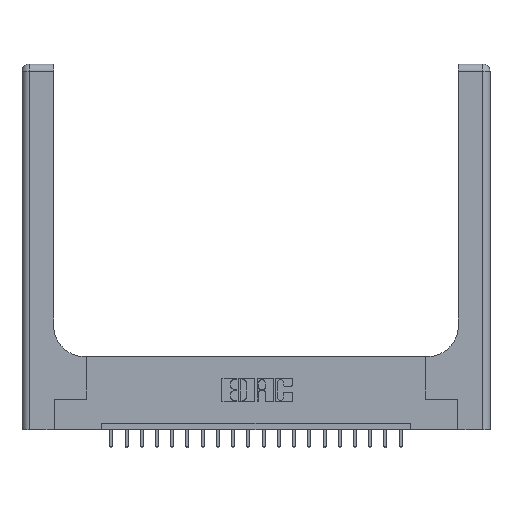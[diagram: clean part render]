
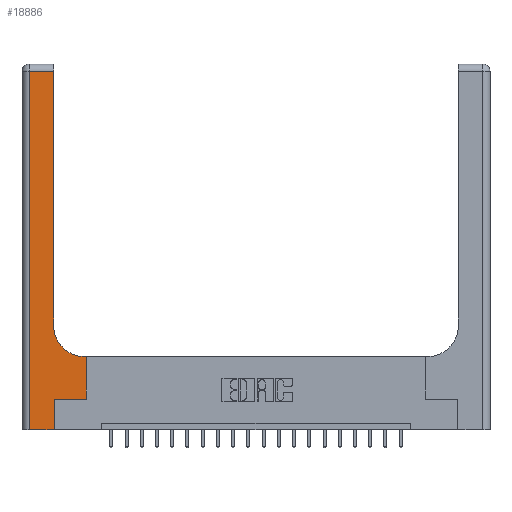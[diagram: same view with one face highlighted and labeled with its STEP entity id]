
A CAD part, top view. The second image highlights one B-rep face of the part: STEP entity #18886.
In plain terms, the highlighted planar face has unit normal (0, 0, 1).
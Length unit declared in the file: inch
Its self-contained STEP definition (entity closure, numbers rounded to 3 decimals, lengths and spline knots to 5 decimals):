
#230 = DIRECTION ( 'NONE',  ( 0., 1., 0. ) ) ;
#360 = CARTESIAN_POINT ( 'NONE',  ( 0.528, 0.25, 0.37 ) ) ;
#778 = VERTEX_POINT ( 'NONE', #14954 ) ;
#841 = DIRECTION ( 'NONE',  ( -1., 0., 0. ) ) ;
#962 = CARTESIAN_POINT ( 'NONE',  ( 0.06, 2.94, 0.37 ) ) ;
#1283 = CARTESIAN_POINT ( 'NONE',  ( 0.26, 0.85, 0.37 ) ) ;
#1516 = ORIENTED_EDGE ( 'NONE', *, *, #11680, .T. ) ;
#2709 = ORIENTED_EDGE ( 'NONE', *, *, #11564, .T. ) ;
#3017 = DIRECTION ( 'NONE',  ( 0., 1., 0. ) ) ;
#3072 = VECTOR ( 'NONE', #16020, 39.37008 ) ;
#3203 = VECTOR ( 'NONE', #3858, 39.37008 ) ;
#3858 = DIRECTION ( 'NONE',  ( 1., 0., 0. ) ) ;
#3915 = CARTESIAN_POINT ( 'NONE',  ( 0.528, 0.25, 0.37 ) ) ;
#4223 = CARTESIAN_POINT ( 'NONE',  ( 0.51, 0.6, 0.37 ) ) ;
#4250 = VERTEX_POINT ( 'NONE', #11984 ) ;
#5029 = DIRECTION ( 'NONE',  ( 0., -1., 0. ) ) ;
#6157 = LINE ( 'NONE', #360, #13315 ) ;
#6390 = VERTEX_POINT ( 'NONE', #7129 ) ;
#6578 = EDGE_CURVE ( 'NONE', #778, #15847, #7678, .T. ) ;
#6653 = CARTESIAN_POINT ( 'NONE',  ( 0.06, 3., 0.37 ) ) ;
#6901 = EDGE_CURVE ( 'NONE', #19575, #14917, #12826, .T. ) ;
#7124 = VECTOR ( 'NONE', #17889, 39.37008 ) ;
#7129 = CARTESIAN_POINT ( 'NONE',  ( 0.265, 0., 0.37 ) ) ;
#7236 = DIRECTION ( 'NONE',  ( 0., 0., -1. ) ) ;
#7390 = AXIS2_PLACEMENT_3D ( 'NONE', #13699, #7236, #7747 ) ;
#7492 = CARTESIAN_POINT ( 'NONE',  ( 0.265, 0., 0.37 ) ) ;
#7678 = LINE ( 'NONE', #18283, #3203 ) ;
#7747 = DIRECTION ( 'NONE',  ( 1., 0., 0. ) ) ;
#8432 = DIRECTION ( 'NONE',  ( 1., 0., 0. ) ) ;
#8637 = CARTESIAN_POINT ( 'NONE',  ( 0., 3., 0.37 ) ) ;
#8917 = EDGE_CURVE ( 'NONE', #13680, #4250, #11285, .T. ) ;
#9224 = VERTEX_POINT ( 'NONE', #9967 ) ;
#9354 = ORIENTED_EDGE ( 'NONE', *, *, #14168, .T. ) ;
#9626 = CARTESIAN_POINT ( 'NONE',  ( 0.26, 2.94, 0.37 ) ) ;
#9837 = ORIENTED_EDGE ( 'NONE', *, *, #8917, .T. ) ;
#9905 = ORIENTED_EDGE ( 'NONE', *, *, #17440, .T. ) ;
#9967 = CARTESIAN_POINT ( 'NONE',  ( 0.528, 0.6, 0.37 ) ) ;
#10087 = LINE ( 'NONE', #14946, #15532 ) ;
#10272 = ORIENTED_EDGE ( 'NONE', *, *, #12328, .T. ) ;
#10383 = DIRECTION ( 'NONE',  ( 0., 0., -1. ) ) ;
#11285 = LINE ( 'NONE', #6653, #20509 ) ;
#11452 = ORIENTED_EDGE ( 'NONE', *, *, #6901, .T. ) ;
#11564 = EDGE_CURVE ( 'NONE', #6390, #778, #12114, .T. ) ;
#11675 = PLANE ( 'NONE',  #18309 ) ;
#11680 = EDGE_CURVE ( 'NONE', #15847, #9224, #6157, .T. ) ;
#11927 = CIRCLE ( 'NONE', #7390, 0.25 ) ;
#11984 = CARTESIAN_POINT ( 'NONE',  ( 0.06, 0., 0.37 ) ) ;
#12114 = LINE ( 'NONE', #7492, #7124 ) ;
#12231 = EDGE_LOOP ( 'NONE', ( #11452, #9354, #9837, #10272, #2709, #13361, #1516, #9905, #14223 ) ) ;
#12328 = EDGE_CURVE ( 'NONE', #4250, #6390, #10087, .T. ) ;
#12357 = VECTOR ( 'NONE', #3017, 39.37008 ) ;
#12713 = LINE ( 'NONE', #20363, #3072 ) ;
#12826 = LINE ( 'NONE', #18957, #12357 ) ;
#12957 = LINE ( 'NONE', #13297, #13450 ) ;
#13297 = CARTESIAN_POINT ( 'NONE',  ( 0.26, 0.6, 0.37 ) ) ;
#13315 = VECTOR ( 'NONE', #230, 39.37008 ) ;
#13361 = ORIENTED_EDGE ( 'NONE', *, *, #6578, .T. ) ;
#13450 = VECTOR ( 'NONE', #841, 39.37008 ) ;
#13680 = VERTEX_POINT ( 'NONE', #962 ) ;
#13699 = CARTESIAN_POINT ( 'NONE',  ( 0.51, 0.85, 0.37 ) ) ;
#14168 = EDGE_CURVE ( 'NONE', #14917, #13680, #12713, .T. ) ;
#14223 = ORIENTED_EDGE ( 'NONE', *, *, #18960, .T. ) ;
#14917 = VERTEX_POINT ( 'NONE', #9626 ) ;
#14946 = CARTESIAN_POINT ( 'NONE',  ( 0., 0., 0.37 ) ) ;
#14954 = CARTESIAN_POINT ( 'NONE',  ( 0.265, 0.25, 0.37 ) ) ;
#15361 = VERTEX_POINT ( 'NONE', #4223 ) ;
#15532 = VECTOR ( 'NONE', #8432, 39.37008 ) ;
#15847 = VERTEX_POINT ( 'NONE', #3915 ) ;
#16020 = DIRECTION ( 'NONE',  ( -1., 0., 0. ) ) ;
#16522 = DIRECTION ( 'NONE',  ( -1., 0., 0. ) ) ;
#17440 = EDGE_CURVE ( 'NONE', #9224, #15361, #12957, .T. ) ;
#17889 = DIRECTION ( 'NONE',  ( 0., 1., 0. ) ) ;
#18283 = CARTESIAN_POINT ( 'NONE',  ( 0.265, 0.25, 0.37 ) ) ;
#18309 = AXIS2_PLACEMENT_3D ( 'NONE', #8637, #10383, #16522 ) ;
#18886 = ADVANCED_FACE ( 'NONE', ( #20373 ), #11675, .F. ) ;
#18957 = CARTESIAN_POINT ( 'NONE',  ( 0.26, 3., 0.37 ) ) ;
#18960 = EDGE_CURVE ( 'NONE', #15361, #19575, #11927, .T. ) ;
#19575 = VERTEX_POINT ( 'NONE', #1283 ) ;
#20363 = CARTESIAN_POINT ( 'NONE',  ( 0., 2.94, 0.37 ) ) ;
#20373 = FACE_OUTER_BOUND ( 'NONE', #12231, .T. ) ;
#20509 = VECTOR ( 'NONE', #5029, 39.37008 ) ;
